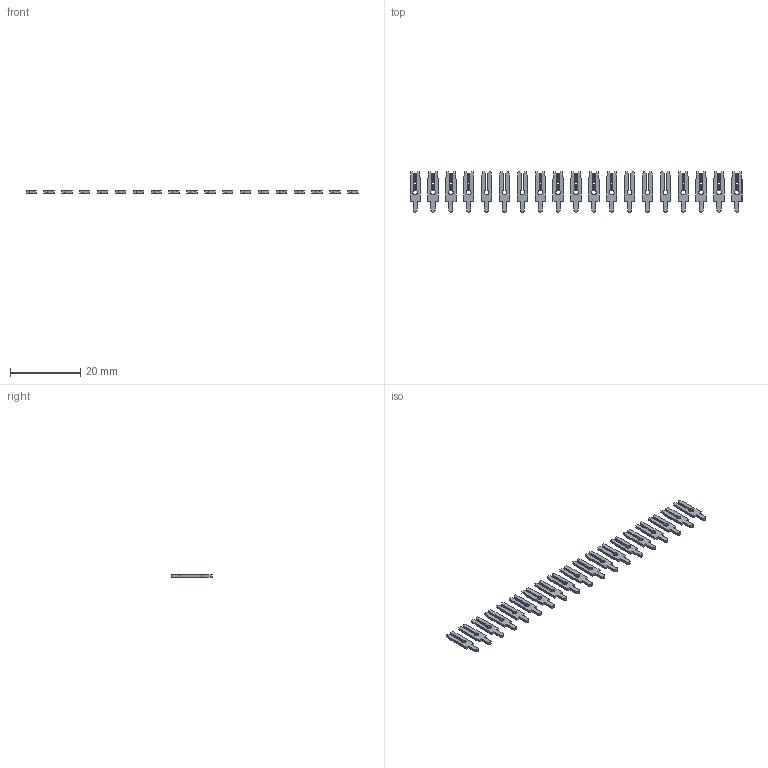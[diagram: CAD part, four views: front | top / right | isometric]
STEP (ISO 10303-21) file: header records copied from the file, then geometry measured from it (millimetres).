
FILE_DESCRIPTION (( 'STEP AP203' ), '1' );
FILE_NAME ('103-019-250-200.STEP', '2020-04-09T20:29:55', ( '' ), ( '' ), 'SwSTEP 2.0', 'SolidWorks 2016', '' );
FILE_SCHEMA (( 'CONFIG_CONTROL_DESIGN' ));
Length unit declared in the file: inch
Products named in the file (2): 103-019-250-200; 100-290-001_100-290-250
Assembly tree (19 placements, depth 2):
  103-019-250-200
    100-290-001_100-290-250  x19
Bounding box: 94.36 x 11.48 x 0.66 mm (x, y, z)
Volume: 296.5 mm3; surface area: 1393.6 mm2
Topology: 19 solids, 19 shells, 456 faces, 1254 edges, 836 vertices
Faces by surface type: plane 380, cylinder 76
Entity records: 1534 total; most frequent: CARTESIAN_POINT 168, DIRECTION 162, ORIENTED_EDGE 132, EDGE_CURVE 66, LINE 54, AXIS2_PLACEMENT_3D 54, VECTOR 54, DATE_AND_TIME 48
